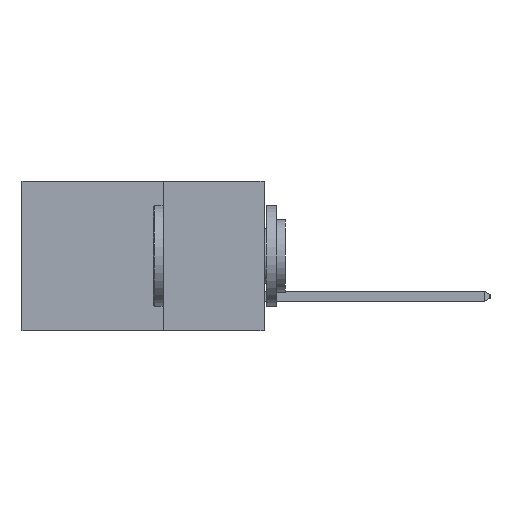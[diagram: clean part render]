
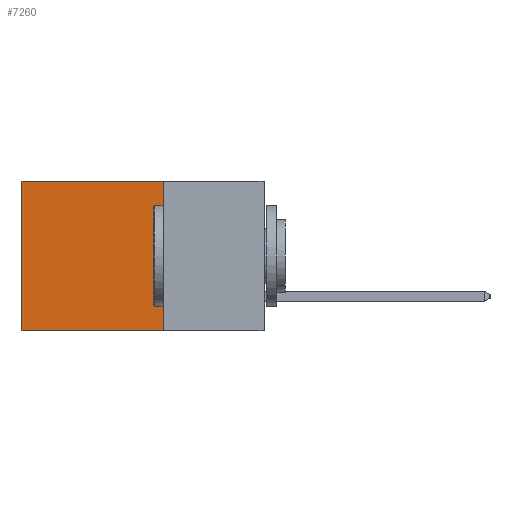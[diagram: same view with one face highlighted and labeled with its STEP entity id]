
A CAD part, left-side view. The second image highlights one B-rep face of the part: STEP entity #7260.
In plain terms, the highlighted planar face has unit normal (-1, 0, 0).
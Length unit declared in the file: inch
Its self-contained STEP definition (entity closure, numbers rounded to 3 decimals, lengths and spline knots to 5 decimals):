
#827 = ORIENTED_EDGE ( 'NONE', *, *, #3100, .T. ) ;
#1503 = FACE_OUTER_BOUND ( 'NONE', #14350, .T. ) ;
#1504 = DIRECTION ( 'NONE',  ( 0., 0., -1. ) ) ;
#1561 = LINE ( 'NONE', #7929, #4488 ) ;
#1588 = CARTESIAN_POINT ( 'NONE',  ( 0.298, 0.6, 0. ) ) ;
#1791 = DIRECTION ( 'NONE',  ( 1., 0., 0. ) ) ;
#2697 = CARTESIAN_POINT ( 'NONE',  ( 0.298, 0.6, 0. ) ) ;
#3100 = EDGE_CURVE ( 'NONE', #13061, #11790, #5712, .T. ) ;
#3800 = CARTESIAN_POINT ( 'NONE',  ( 0.298, 0.25, 0. ) ) ;
#4488 = VECTOR ( 'NONE', #11648, 39.37008 ) ;
#4552 = AXIS2_PLACEMENT_3D ( 'NONE', #13711, #1791, #1504 ) ;
#4630 = LINE ( 'NONE', #1588, #4999 ) ;
#4999 = VECTOR ( 'NONE', #13195, 39.37008 ) ;
#5383 = DIRECTION ( 'NONE',  ( 0., 1., 0. ) ) ;
#5712 = LINE ( 'NONE', #14334, #15424 ) ;
#6721 = CARTESIAN_POINT ( 'NONE',  ( 0.298, 0.6, -0.37 ) ) ;
#7080 = EDGE_CURVE ( 'NONE', #11790, #7224, #4630, .T. ) ;
#7224 = VERTEX_POINT ( 'NONE', #6721 ) ;
#7260 = ADVANCED_FACE ( 'NONE', ( #1503 ), #8334, .F. ) ;
#7929 = CARTESIAN_POINT ( 'NONE',  ( 0.298, 0.25, -0.37 ) ) ;
#8334 = PLANE ( 'NONE',  #4552 ) ;
#8534 = CARTESIAN_POINT ( 'NONE',  ( 0.298, 0.25, 0. ) ) ;
#8587 = VECTOR ( 'NONE', #14796, 39.37008 ) ;
#8747 = CARTESIAN_POINT ( 'NONE',  ( 0.298, 0.25, -0.37 ) ) ;
#10430 = VERTEX_POINT ( 'NONE', #8747 ) ;
#10648 = ORIENTED_EDGE ( 'NONE', *, *, #7080, .T. ) ;
#10653 = ORIENTED_EDGE ( 'NONE', *, *, #13997, .F. ) ;
#11648 = DIRECTION ( 'NONE',  ( 0., 1., 0. ) ) ;
#11790 = VERTEX_POINT ( 'NONE', #2697 ) ;
#13061 = VERTEX_POINT ( 'NONE', #8534 ) ;
#13195 = DIRECTION ( 'NONE',  ( 0., 0., -1. ) ) ;
#13711 = CARTESIAN_POINT ( 'NONE',  ( 0.298, 0.25, 0. ) ) ;
#13848 = ORIENTED_EDGE ( 'NONE', *, *, #14762, .F. ) ;
#13997 = EDGE_CURVE ( 'NONE', #13061, #10430, #14681, .T. ) ;
#14334 = CARTESIAN_POINT ( 'NONE',  ( 0.298, 0.25, 0. ) ) ;
#14350 = EDGE_LOOP ( 'NONE', ( #10648, #13848, #10653, #827 ) ) ;
#14681 = LINE ( 'NONE', #3800, #8587 ) ;
#14762 = EDGE_CURVE ( 'NONE', #10430, #7224, #1561, .T. ) ;
#14796 = DIRECTION ( 'NONE',  ( 0., 0., -1. ) ) ;
#15424 = VECTOR ( 'NONE', #5383, 39.37008 ) ;
